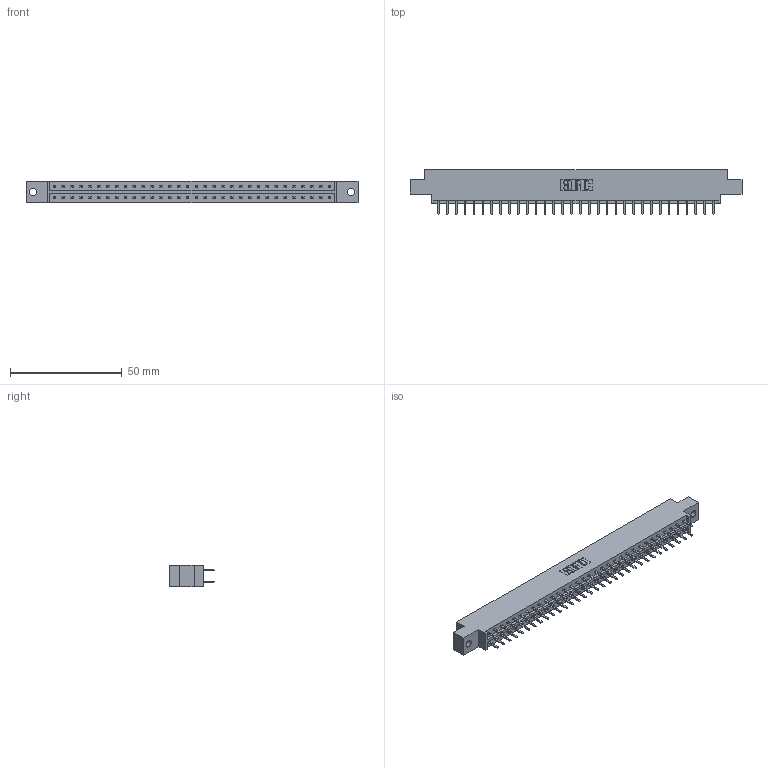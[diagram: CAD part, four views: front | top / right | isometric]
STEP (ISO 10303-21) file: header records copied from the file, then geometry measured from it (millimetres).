
FILE_DESCRIPTION (( 'STEP AP203' ), '1' );
FILE_NAME ('333-064-520-802.STEP', '2018-08-04T09:28:57', ( '' ), ( '' ), 'SwSTEP 2.0', 'SolidWorks 2016', '' );
FILE_SCHEMA (( 'CONFIG_CONTROL_DESIGN' ));
Length unit declared in the file: inch
Products named in the file (3): 345-292-001_345-293-120; 333-064-520-802; 333 Part_Offset - .128 Dia
Assembly tree (65 placements, depth 2):
  333-064-520-802
    333 Part_Offset - .128 Dia
    345-292-001_345-293-120  x64
Bounding box: 148.34 x 20.02 x 9.4 mm (x, y, z)
Volume: 14758.1 mm3; surface area: 17213.3 mm2
Topology: 65 solids, 65 shells, 3702 faces, 10755 edges, 6998 vertices
Faces by surface type: plane 2506, cylinder 1196
Entity records: 22129 total; most frequent: CARTESIAN_POINT 3694, ORIENTED_EDGE 3618, DIRECTION 3161, EDGE_CURVE 1809, LINE 1677, VECTOR 1677, VERTEX_POINT 1202, AXIS2_PLACEMENT_3D 742
